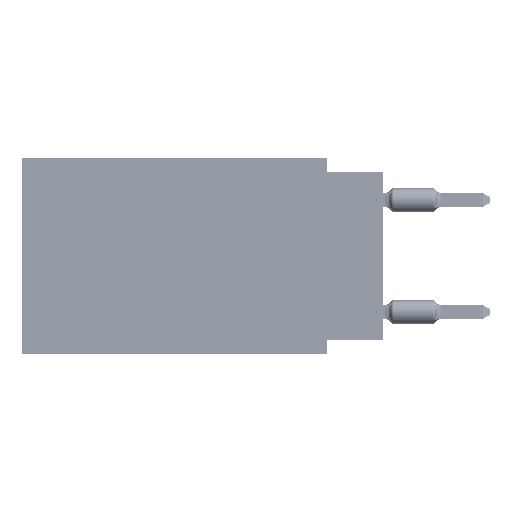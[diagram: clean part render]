
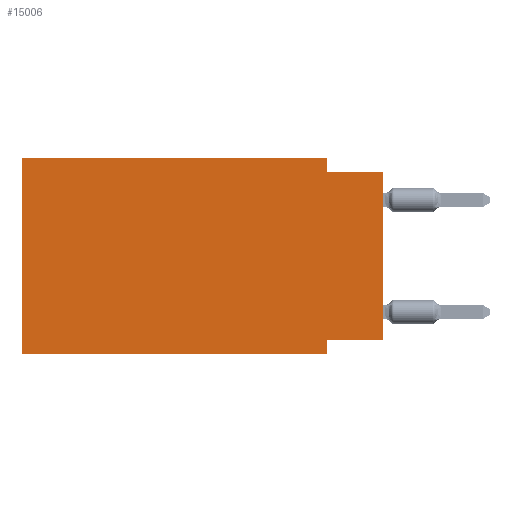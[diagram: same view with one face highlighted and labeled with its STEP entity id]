
A CAD part, left-side view. The second image highlights one B-rep face of the part: STEP entity #15006.
In plain terms, the highlighted planar face has unit normal (-1, 0, 0).
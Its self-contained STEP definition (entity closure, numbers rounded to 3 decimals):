
#245 = DIRECTION ( 'NONE',  ( 0., -1., 0. ) ) ;
#822 = CARTESIAN_POINT ( 'NONE',  ( 0., 16.383, 0. ) ) ;
#1180 = LINE ( 'NONE', #5333, #21057 ) ;
#2141 = VERTEX_POINT ( 'NONE', #9463 ) ;
#2409 = DIRECTION ( 'NONE',  ( 0., -1., 0. ) ) ;
#4836 = CARTESIAN_POINT ( 'NONE',  ( 0., 2.54, -0.635 ) ) ;
#5150 = DIRECTION ( 'NONE',  ( 0., 0., 1. ) ) ;
#5333 = CARTESIAN_POINT ( 'NONE',  ( 0., 0., -0.635 ) ) ;
#6292 = CARTESIAN_POINT ( 'NONE',  ( 0., 16.383, 0. ) ) ;
#6583 = VERTEX_POINT ( 'NONE', #42290 ) ;
#7882 = EDGE_CURVE ( 'NONE', #29552, #18551, #45606, .T. ) ;
#9463 = CARTESIAN_POINT ( 'NONE',  ( 0., 0., -0.635 ) ) ;
#10413 = ORIENTED_EDGE ( 'NONE', *, *, #12904, .F. ) ;
#10717 = EDGE_LOOP ( 'NONE', ( #50524, #21461, #55955, #12856, #10413, #19347, #35185, #42603 ) ) ;
#10986 = VECTOR ( 'NONE', #245, 1000. ) ;
#11318 = CARTESIAN_POINT ( 'NONE',  ( 0., 16.383, -8.89 ) ) ;
#12514 = DIRECTION ( 'NONE',  ( 0., 0., -1. ) ) ;
#12856 = ORIENTED_EDGE ( 'NONE', *, *, #7882, .F. ) ;
#12904 = EDGE_CURVE ( 'NONE', #56459, #29552, #51973, .T. ) ;
#14091 = FACE_OUTER_BOUND ( 'NONE', #10717, .T. ) ;
#14229 = DIRECTION ( 'NONE',  ( 0., -1., 0. ) ) ;
#15006 = ADVANCED_FACE ( 'NONE', ( #14091 ), #53852, .F. ) ;
#15219 = LINE ( 'NONE', #23833, #24117 ) ;
#17123 = CARTESIAN_POINT ( 'NONE',  ( 0., 2.54, 0. ) ) ;
#17268 = CARTESIAN_POINT ( 'NONE',  ( 0., 0., -8.255 ) ) ;
#17998 = EDGE_CURVE ( 'NONE', #18320, #2141, #15219, .T. ) ;
#18320 = VERTEX_POINT ( 'NONE', #17268 ) ;
#18551 = VERTEX_POINT ( 'NONE', #17123 ) ;
#19347 = ORIENTED_EDGE ( 'NONE', *, *, #30032, .T. ) ;
#21057 = VECTOR ( 'NONE', #14229, 1000. ) ;
#21082 = LINE ( 'NONE', #11318, #28372 ) ;
#21461 = ORIENTED_EDGE ( 'NONE', *, *, #45735, .F. ) ;
#22428 = VECTOR ( 'NONE', #43650, 1000. ) ;
#22744 = EDGE_CURVE ( 'NONE', #18320, #37818, #29712, .T. ) ;
#23833 = CARTESIAN_POINT ( 'NONE',  ( 0., 0., 0. ) ) ;
#24117 = VECTOR ( 'NONE', #5150, 1000. ) ;
#24816 = VECTOR ( 'NONE', #37461, 1000. ) ;
#28050 = DIRECTION ( 'NONE',  ( 0., 0., -1. ) ) ;
#28162 = VERTEX_POINT ( 'NONE', #4836 ) ;
#28372 = VECTOR ( 'NONE', #2409, 1000. ) ;
#29552 = VERTEX_POINT ( 'NONE', #822 ) ;
#29712 = LINE ( 'NONE', #49270, #22428 ) ;
#30032 = EDGE_CURVE ( 'NONE', #56459, #6583, #21082, .T. ) ;
#30605 = LINE ( 'NONE', #35656, #32710 ) ;
#30839 = VECTOR ( 'NONE', #28050, 1000. ) ;
#31908 = CARTESIAN_POINT ( 'NONE',  ( 0., 2.54, -8.89 ) ) ;
#32178 = CARTESIAN_POINT ( 'NONE',  ( 0., 16.383, 0. ) ) ;
#32710 = VECTOR ( 'NONE', #12514, 1000. ) ;
#35185 = ORIENTED_EDGE ( 'NONE', *, *, #51658, .F. ) ;
#35656 = CARTESIAN_POINT ( 'NONE',  ( 0., 2.54, 0. ) ) ;
#36676 = CARTESIAN_POINT ( 'NONE',  ( 0., 2.54, -8.255 ) ) ;
#37461 = DIRECTION ( 'NONE',  ( 0., 0., 1. ) ) ;
#37818 = VERTEX_POINT ( 'NONE', #36676 ) ;
#38504 = EDGE_CURVE ( 'NONE', #18551, #28162, #30605, .T. ) ;
#41378 = DIRECTION ( 'NONE',  ( 0., 0., -1. ) ) ;
#42290 = CARTESIAN_POINT ( 'NONE',  ( 0., 2.54, -8.89 ) ) ;
#42551 = CARTESIAN_POINT ( 'NONE',  ( 0., 16.383, 0. ) ) ;
#42603 = ORIENTED_EDGE ( 'NONE', *, *, #22744, .F. ) ;
#43650 = DIRECTION ( 'NONE',  ( 0., 1., 0. ) ) ;
#45606 = LINE ( 'NONE', #42551, #10986 ) ;
#45735 = EDGE_CURVE ( 'NONE', #28162, #2141, #1180, .T. ) ;
#45814 = DIRECTION ( 'NONE',  ( 1., 0., 0. ) ) ;
#48582 = CARTESIAN_POINT ( 'NONE',  ( 0., 16.383, -8.89 ) ) ;
#49270 = CARTESIAN_POINT ( 'NONE',  ( 0., 0., -8.255 ) ) ;
#50524 = ORIENTED_EDGE ( 'NONE', *, *, #17998, .T. ) ;
#50595 = LINE ( 'NONE', #31908, #30839 ) ;
#51658 = EDGE_CURVE ( 'NONE', #37818, #6583, #50595, .T. ) ;
#51973 = LINE ( 'NONE', #6292, #24816 ) ;
#53257 = AXIS2_PLACEMENT_3D ( 'NONE', #32178, #45814, #41378 ) ;
#53852 = PLANE ( 'NONE',  #53257 ) ;
#55955 = ORIENTED_EDGE ( 'NONE', *, *, #38504, .F. ) ;
#56459 = VERTEX_POINT ( 'NONE', #48582 ) ;
